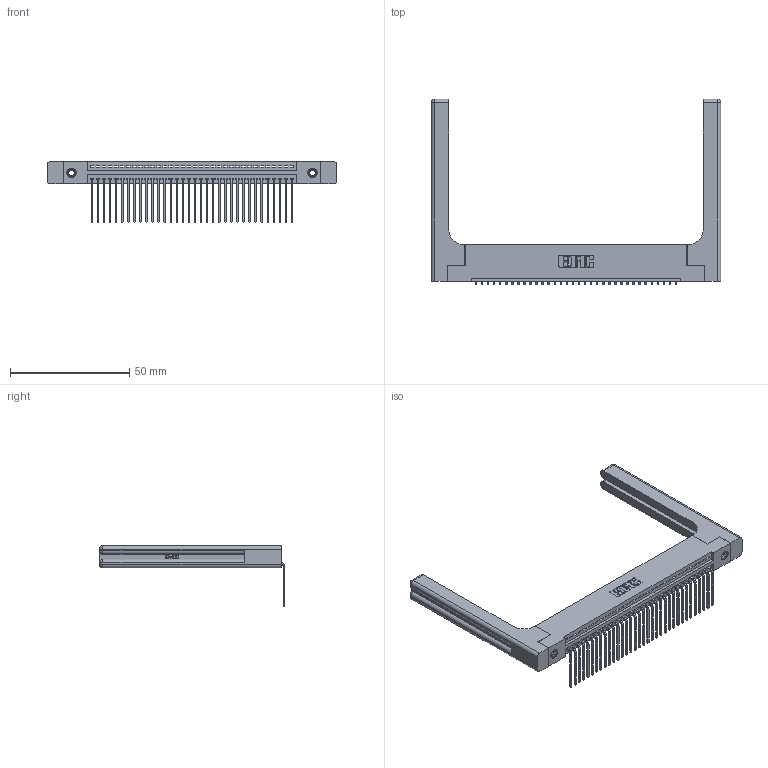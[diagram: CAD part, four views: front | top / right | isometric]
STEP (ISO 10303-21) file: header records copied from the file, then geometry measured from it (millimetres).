
FILE_DESCRIPTION (( 'STEP AP203' ), '1' );
FILE_NAME ('395-034-559-158.STEP', '2019-10-19T18:20:23', ( '' ), ( '' ), 'SwSTEP 2.0', 'SolidWorks 2016', '' );
FILE_SCHEMA (( 'CONFIG_CONTROL_DESIGN' ));
Length unit declared in the file: inch
Products named in the file (5): 395-034-559-158; 345-292-001_558 559 Tail - 1; 345 Part_Flush Mounting Lugs - 0.156 Dia-TH; 345-220-058_345-220-058; 345-250-001_345-250-001-102
Assembly tree (39 placements, depth 2):
  395-034-559-158
    345 Part_Flush Mounting Lugs - 0.156 Dia-TH
    345-292-001_558 559 Tail - 1  x34
    345-250-001_345-250-001-102  x2
    345-220-058_345-220-058  x2
Bounding box: 121.39 x 77.71 x 25.53 mm (x, y, z)
Volume: 20082.1 mm3; surface area: 21247.5 mm2
Topology: 39 solids, 39 shells, 2422 faces, 7195 edges, 4730 vertices
Faces by surface type: plane 1656, cylinder 706, bspline 36, cone 12, sphere 8, torus 4
Entity records: 31932 total; most frequent: CARTESIAN_POINT 6503, ORIENTED_EDGE 5268, DIRECTION 4638, EDGE_CURVE 2634, VECTOR 2274, LINE 2274, VERTEX_POINT 1746, AXIS2_PLACEMENT_3D 1182
